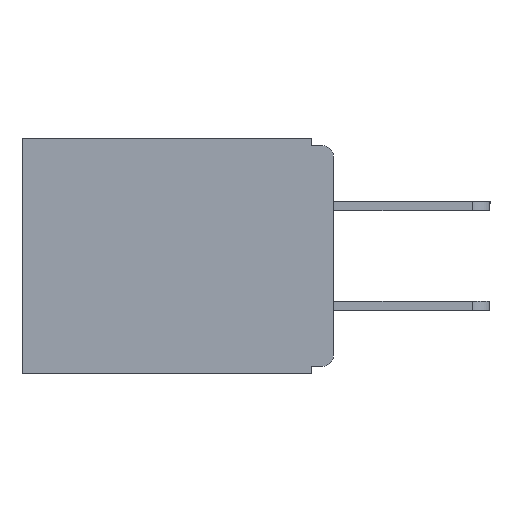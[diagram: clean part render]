
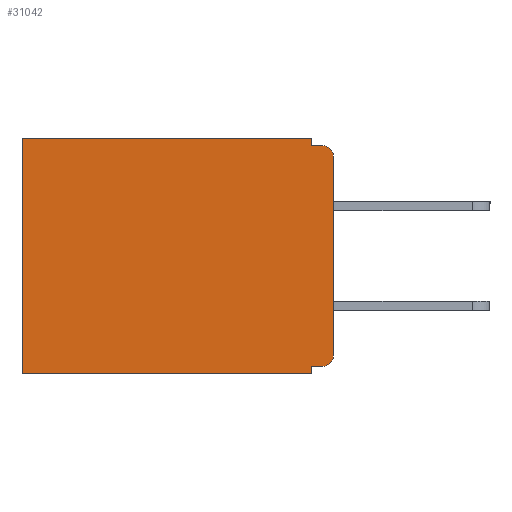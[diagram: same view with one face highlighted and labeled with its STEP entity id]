
A CAD part, left-side view. The second image highlights one B-rep face of the part: STEP entity #31042.
In plain terms, the highlighted planar face has unit normal (-1, 0, 0).
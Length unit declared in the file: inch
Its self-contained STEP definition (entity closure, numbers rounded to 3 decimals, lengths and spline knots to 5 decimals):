
#106 = DIRECTION ( 'NONE',  ( -1., 0., 0. ) ) ;
#1052 = VERTEX_POINT ( 'NONE', #28059 ) ;
#1859 = VERTEX_POINT ( 'NONE', #3844 ) ;
#2242 = VECTOR ( 'NONE', #32126, 39.37008 ) ;
#2396 = LINE ( 'NONE', #28219, #16696 ) ;
#2512 = LINE ( 'NONE', #12673, #29130 ) ;
#3060 = EDGE_CURVE ( 'NONE', #1052, #6355, #8500, .T. ) ;
#3216 = ORIENTED_EDGE ( 'NONE', *, *, #28719, .T. ) ;
#3707 = CARTESIAN_POINT ( 'NONE',  ( 0.3, 0., -0.33 ) ) ;
#3808 = ORIENTED_EDGE ( 'NONE', *, *, #11809, .F. ) ;
#3844 = CARTESIAN_POINT ( 'NONE',  ( 0.3, 0.031, -0.33 ) ) ;
#3970 = VERTEX_POINT ( 'NONE', #26143 ) ;
#4949 = LINE ( 'NONE', #5831, #7462 ) ;
#5245 = CARTESIAN_POINT ( 'NONE',  ( 0.3, 0.437, -0.33 ) ) ;
#5350 = CARTESIAN_POINT ( 'NONE',  ( 0.3, 0., -0.33 ) ) ;
#5465 = ORIENTED_EDGE ( 'NONE', *, *, #15644, .F. ) ;
#5480 = DIRECTION ( 'NONE',  ( 1., 0., 0. ) ) ;
#5831 = CARTESIAN_POINT ( 'NONE',  ( 0.3, 0., 0. ) ) ;
#6271 = VECTOR ( 'NONE', #8103, 39.37008 ) ;
#6355 = VERTEX_POINT ( 'NONE', #18394 ) ;
#6377 = ORIENTED_EDGE ( 'NONE', *, *, #22063, .T. ) ;
#7298 = ORIENTED_EDGE ( 'NONE', *, *, #23774, .T. ) ;
#7416 = VERTEX_POINT ( 'NONE', #18957 ) ;
#7462 = VECTOR ( 'NONE', #8531, 39.37008 ) ;
#7649 = VERTEX_POINT ( 'NONE', #32754 ) ;
#8103 = DIRECTION ( 'NONE',  ( 0., 1., 0. ) ) ;
#8188 = CARTESIAN_POINT ( 'NONE',  ( 0.3, 0.015, -0.32 ) ) ;
#8500 = LINE ( 'NONE', #32799, #2242 ) ;
#8531 = DIRECTION ( 'NONE',  ( 0., 1., 0. ) ) ;
#8828 = EDGE_CURVE ( 'NONE', #1859, #22139, #32879, .T. ) ;
#9394 = VERTEX_POINT ( 'NONE', #14029 ) ;
#9642 = DIRECTION ( 'NONE',  ( 0., 0., -1. ) ) ;
#9960 = VECTOR ( 'NONE', #14790, 39.37008 ) ;
#10691 = CARTESIAN_POINT ( 'NONE',  ( 0.3, 0., -0.32 ) ) ;
#10756 = PLANE ( 'NONE',  #30774 ) ;
#11061 = EDGE_CURVE ( 'NONE', #33124, #3970, #24121, .T. ) ;
#11534 = CIRCLE ( 'NONE', #22563, 0.015 ) ;
#11809 = EDGE_CURVE ( 'NONE', #7416, #1859, #2396, .T. ) ;
#12047 = CARTESIAN_POINT ( 'NONE',  ( 0.3, 0.031, 0. ) ) ;
#12673 = CARTESIAN_POINT ( 'NONE',  ( 0.3, 0., -0.01 ) ) ;
#12849 = EDGE_LOOP ( 'NONE', ( #15766, #6377, #5465, #13994, #7298, #3216, #20586, #3808, #15583, #28735 ) ) ;
#13994 = ORIENTED_EDGE ( 'NONE', *, *, #11061, .F. ) ;
#14029 = CARTESIAN_POINT ( 'NONE',  ( 0.3, 0.437, 0. ) ) ;
#14683 = CARTESIAN_POINT ( 'NONE',  ( 0.3, 0.015, -0.025 ) ) ;
#14790 = DIRECTION ( 'NONE',  ( 0., 0., -1. ) ) ;
#15423 = DIRECTION ( 'NONE',  ( 0., -1., 0. ) ) ;
#15583 = ORIENTED_EDGE ( 'NONE', *, *, #23084, .F. ) ;
#15644 = EDGE_CURVE ( 'NONE', #3970, #7649, #2512, .T. ) ;
#15766 = ORIENTED_EDGE ( 'NONE', *, *, #3060, .F. ) ;
#16288 = CARTESIAN_POINT ( 'NONE',  ( 0.3, 0.015, -0.305 ) ) ;
#16696 = VECTOR ( 'NONE', #9642, 39.37008 ) ;
#17427 = DIRECTION ( 'NONE',  ( 0., 0., -1. ) ) ;
#18394 = CARTESIAN_POINT ( 'NONE',  ( 0.3, 0., -0.305 ) ) ;
#18666 = DIRECTION ( 'NONE',  ( 0., 0., -1. ) ) ;
#18706 = EDGE_CURVE ( 'NONE', #19305, #6355, #11534, .T. ) ;
#18955 = DIRECTION ( 'NONE',  ( 0., 0., -1. ) ) ;
#18957 = CARTESIAN_POINT ( 'NONE',  ( 0.3, 0.031, -0.32 ) ) ;
#19305 = VERTEX_POINT ( 'NONE', #8188 ) ;
#20249 = CARTESIAN_POINT ( 'NONE',  ( 0.3, 0.437, -0.33 ) ) ;
#20380 = VECTOR ( 'NONE', #18666, 39.37008 ) ;
#20586 = ORIENTED_EDGE ( 'NONE', *, *, #8828, .F. ) ;
#21185 = LINE ( 'NONE', #5245, #20380 ) ;
#22063 = EDGE_CURVE ( 'NONE', #1052, #7649, #30396, .T. ) ;
#22139 = VERTEX_POINT ( 'NONE', #20249 ) ;
#22383 = DIRECTION ( 'NONE',  ( 0., 1., 0. ) ) ;
#22563 = AXIS2_PLACEMENT_3D ( 'NONE', #16288, #106, #18955 ) ;
#22740 = CARTESIAN_POINT ( 'NONE',  ( 0.3, 0.031, 0. ) ) ;
#23084 = EDGE_CURVE ( 'NONE', #19305, #7416, #34409, .T. ) ;
#23519 = FACE_OUTER_BOUND ( 'NONE', #12849, .T. ) ;
#23774 = EDGE_CURVE ( 'NONE', #33124, #9394, #4949, .T. ) ;
#24121 = LINE ( 'NONE', #12047, #9960 ) ;
#24130 = DIRECTION ( 'NONE',  ( 0., 0., -1. ) ) ;
#25097 = VECTOR ( 'NONE', #22383, 39.37008 ) ;
#26143 = CARTESIAN_POINT ( 'NONE',  ( 0.3, 0.031, -0.01 ) ) ;
#28059 = CARTESIAN_POINT ( 'NONE',  ( 0.3, 0., -0.025 ) ) ;
#28219 = CARTESIAN_POINT ( 'NONE',  ( 0.3, 0.031, -0.33 ) ) ;
#28719 = EDGE_CURVE ( 'NONE', #9394, #22139, #21185, .T. ) ;
#28735 = ORIENTED_EDGE ( 'NONE', *, *, #18706, .T. ) ;
#29130 = VECTOR ( 'NONE', #15423, 39.37008 ) ;
#29927 = AXIS2_PLACEMENT_3D ( 'NONE', #14683, #33056, #17427 ) ;
#30396 = CIRCLE ( 'NONE', #29927, 0.015 ) ;
#30774 = AXIS2_PLACEMENT_3D ( 'NONE', #5350, #5480, #24130 ) ;
#31042 = ADVANCED_FACE ( 'NONE', ( #23519 ), #10756, .F. ) ;
#32126 = DIRECTION ( 'NONE',  ( 0., 0., -1. ) ) ;
#32754 = CARTESIAN_POINT ( 'NONE',  ( 0.3, 0.015, -0.01 ) ) ;
#32799 = CARTESIAN_POINT ( 'NONE',  ( 0.3, 0., -0.33 ) ) ;
#32879 = LINE ( 'NONE', #3707, #25097 ) ;
#33056 = DIRECTION ( 'NONE',  ( -1., 0., 0. ) ) ;
#33124 = VERTEX_POINT ( 'NONE', #22740 ) ;
#34409 = LINE ( 'NONE', #10691, #6271 ) ;
